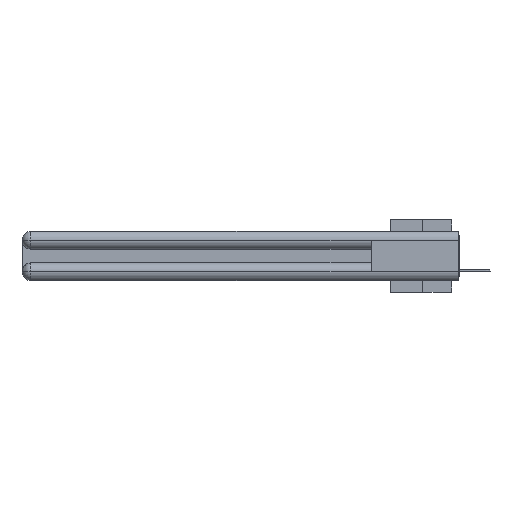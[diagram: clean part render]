
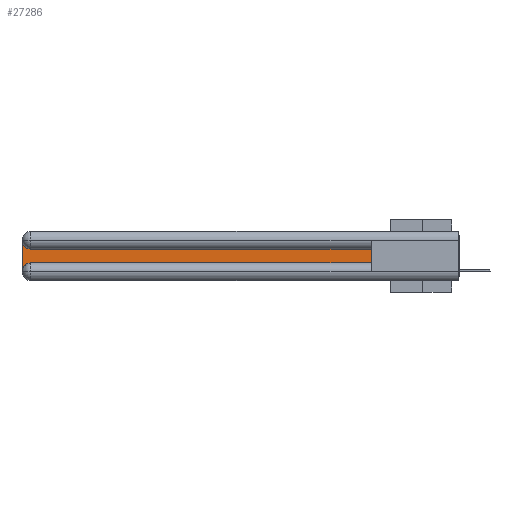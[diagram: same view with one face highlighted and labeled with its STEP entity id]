
A CAD part, left-side view. The second image highlights one B-rep face of the part: STEP entity #27286.
In plain terms, the highlighted planar face has unit normal (-1, 0, 0).
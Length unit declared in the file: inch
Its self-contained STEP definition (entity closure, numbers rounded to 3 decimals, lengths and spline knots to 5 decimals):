
#516 = ORIENTED_EDGE ( 'NONE', *, *, #886, .T. ) ;
#886 = EDGE_CURVE ( 'NONE', #1059, #11219, #10485, .T. ) ;
#973 = FACE_OUTER_BOUND ( 'NONE', #11721, .T. ) ;
#1059 = VERTEX_POINT ( 'NONE', #3050 ) ;
#2420 = DIRECTION ( 'NONE',  ( 0., 0., 1. ) ) ;
#2495 = DIRECTION ( 'NONE',  ( 0., -1., 0. ) ) ;
#2618 = CARTESIAN_POINT ( 'NONE',  ( 0.075, 0.6, -0.1225 ) ) ;
#3050 = CARTESIAN_POINT ( 'NONE',  ( 0.075, 2.94, -0.1225 ) ) ;
#4285 = DIRECTION ( 'NONE',  ( 0., 0., -1. ) ) ;
#4326 = LINE ( 'NONE', #20492, #28622 ) ;
#5118 = CARTESIAN_POINT ( 'NONE',  ( 0.075, 0.6, -0.2175 ) ) ;
#5329 = ORIENTED_EDGE ( 'NONE', *, *, #9178, .T. ) ;
#5655 = AXIS2_PLACEMENT_3D ( 'NONE', #10341, #17283, #4285 ) ;
#5788 = ORIENTED_EDGE ( 'NONE', *, *, #8760, .T. ) ;
#6264 = DIRECTION ( 'NONE',  ( 0., 0., -1. ) ) ;
#6528 = CARTESIAN_POINT ( 'NONE',  ( 0.075, 2.94, -0.2775 ) ) ;
#6946 = VECTOR ( 'NONE', #25291, 39.37008 ) ;
#7014 = ORIENTED_EDGE ( 'NONE', *, *, #23123, .T. ) ;
#8760 = EDGE_CURVE ( 'NONE', #12222, #13157, #23569, .T. ) ;
#9178 = EDGE_CURVE ( 'NONE', #16647, #12222, #4326, .T. ) ;
#9252 = DIRECTION ( 'NONE',  ( 0., 0., -1. ) ) ;
#9731 = LINE ( 'NONE', #2618, #6946 ) ;
#10341 = CARTESIAN_POINT ( 'NONE',  ( 0.075, 2.94, -0.0625 ) ) ;
#10485 = CIRCLE ( 'NONE', #5655, 0.06 ) ;
#10502 = LINE ( 'NONE', #17752, #15980 ) ;
#10519 = ORIENTED_EDGE ( 'NONE', *, *, #22585, .T. ) ;
#11219 = VERTEX_POINT ( 'NONE', #21947 ) ;
#11721 = EDGE_LOOP ( 'NONE', ( #11874, #516, #10519, #7014, #5329, #5788 ) ) ;
#11874 = ORIENTED_EDGE ( 'NONE', *, *, #12756, .T. ) ;
#12222 = VERTEX_POINT ( 'NONE', #25045 ) ;
#12319 = DIRECTION ( 'NONE',  ( 0., 0., -1. ) ) ;
#12756 = EDGE_CURVE ( 'NONE', #13157, #1059, #9731, .T. ) ;
#13157 = VERTEX_POINT ( 'NONE', #19707 ) ;
#13449 = CARTESIAN_POINT ( 'NONE',  ( 0.075, 2.94, -0.2175 ) ) ;
#13779 = DIRECTION ( 'NONE',  ( 1., 0., 0. ) ) ;
#14040 = VERTEX_POINT ( 'NONE', #22007 ) ;
#15980 = VECTOR ( 'NONE', #6264, 39.37008 ) ;
#16647 = VERTEX_POINT ( 'NONE', #13449 ) ;
#17283 = DIRECTION ( 'NONE',  ( 1., 0., 0. ) ) ;
#17752 = CARTESIAN_POINT ( 'NONE',  ( 0.075, 3., -0.2175 ) ) ;
#18664 = CARTESIAN_POINT ( 'NONE',  ( 0.075, 3., -0.1225 ) ) ;
#19707 = CARTESIAN_POINT ( 'NONE',  ( 0.075, 0.6, -0.1225 ) ) ;
#20492 = CARTESIAN_POINT ( 'NONE',  ( 0.075, 0.6, -0.2175 ) ) ;
#21688 = CIRCLE ( 'NONE', #27000, 0.06 ) ;
#21947 = CARTESIAN_POINT ( 'NONE',  ( 0.075, 3., -0.0625 ) ) ;
#22007 = CARTESIAN_POINT ( 'NONE',  ( 0.075, 3., -0.2775 ) ) ;
#22585 = EDGE_CURVE ( 'NONE', #11219, #14040, #10502, .T. ) ;
#23123 = EDGE_CURVE ( 'NONE', #14040, #16647, #21688, .T. ) ;
#23569 = LINE ( 'NONE', #5118, #29099 ) ;
#25045 = CARTESIAN_POINT ( 'NONE',  ( 0.075, 0.6, -0.2175 ) ) ;
#25291 = DIRECTION ( 'NONE',  ( 0., 1., 0. ) ) ;
#25909 = DIRECTION ( 'NONE',  ( 1., 0., 0. ) ) ;
#27000 = AXIS2_PLACEMENT_3D ( 'NONE', #6528, #13779, #9252 ) ;
#27286 = ADVANCED_FACE ( 'NONE', ( #973 ), #28350, .F. ) ;
#28259 = AXIS2_PLACEMENT_3D ( 'NONE', #18664, #25909, #12319 ) ;
#28350 = PLANE ( 'NONE',  #28259 ) ;
#28622 = VECTOR ( 'NONE', #2495, 39.37008 ) ;
#29099 = VECTOR ( 'NONE', #2420, 39.37008 ) ;
